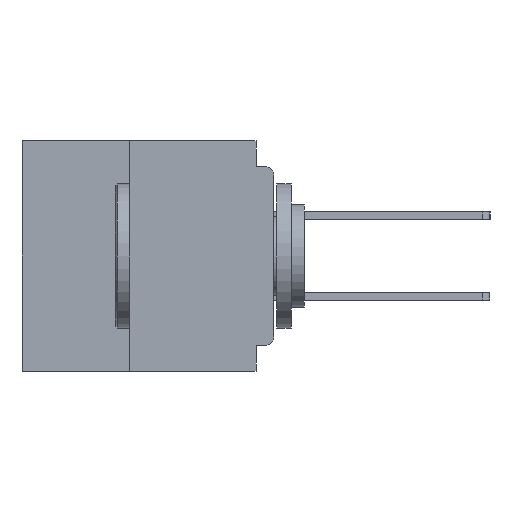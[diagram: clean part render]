
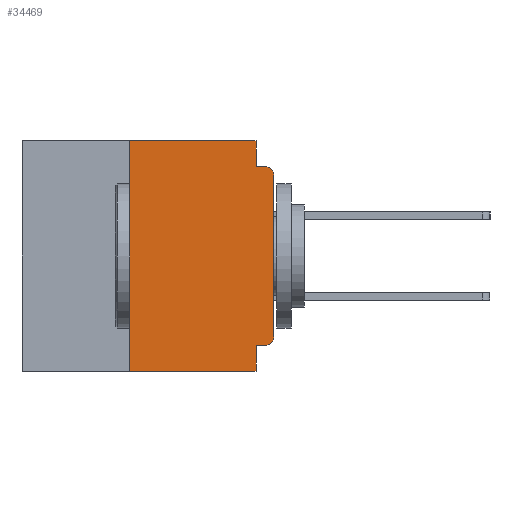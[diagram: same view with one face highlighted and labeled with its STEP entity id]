
A CAD part, left-side view. The second image highlights one B-rep face of the part: STEP entity #34469.
In plain terms, the highlighted planar face has unit normal (-1, 0, 0).
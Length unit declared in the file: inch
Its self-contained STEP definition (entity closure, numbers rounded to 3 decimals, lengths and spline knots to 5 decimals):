
#157 = ORIENTED_EDGE ( 'NONE', *, *, #12103, .T. ) ;
#930 = PLANE ( 'NONE',  #47290 ) ;
#1720 = LINE ( 'NONE', #28280, #22312 ) ;
#2714 = CARTESIAN_POINT ( 'NONE',  ( 0., 0.015, -0.34 ) ) ;
#3421 = CARTESIAN_POINT ( 'NONE',  ( 0., 0., -0.355 ) ) ;
#5037 = DIRECTION ( 'NONE',  ( 1., 0., 0. ) ) ;
#6052 = CARTESIAN_POINT ( 'NONE',  ( 0., 0.015, -0.06 ) ) ;
#6749 = EDGE_CURVE ( 'NONE', #33554, #48301, #14024, .T. ) ;
#6800 = DIRECTION ( 'NONE',  ( 0., 0., -1. ) ) ;
#7223 = CIRCLE ( 'NONE', #9165, 0.015 ) ;
#7630 = LINE ( 'NONE', #3421, #28279 ) ;
#8151 = CARTESIAN_POINT ( 'NONE',  ( 0., 0.031, -0.355 ) ) ;
#8238 = ORIENTED_EDGE ( 'NONE', *, *, #46837, .T. ) ;
#9165 = AXIS2_PLACEMENT_3D ( 'NONE', #6052, #34853, #10211 ) ;
#9646 = LINE ( 'NONE', #21950, #41076 ) ;
#10211 = DIRECTION ( 'NONE',  ( 0., 0., -1. ) ) ;
#10307 = EDGE_CURVE ( 'NONE', #15700, #12959, #27178, .T. ) ;
#10520 = CARTESIAN_POINT ( 'NONE',  ( 0., 0., 0. ) ) ;
#11860 = CARTESIAN_POINT ( 'NONE',  ( 0., 0.015, -0.045 ) ) ;
#12103 = EDGE_CURVE ( 'NONE', #51510, #29563, #7223, .T. ) ;
#12351 = CARTESIAN_POINT ( 'NONE',  ( 0., 0.25, 0. ) ) ;
#12959 = VERTEX_POINT ( 'NONE', #40966 ) ;
#13499 = LINE ( 'NONE', #20891, #43591 ) ;
#13823 = CARTESIAN_POINT ( 'NONE',  ( 0., 0.437, -0.4 ) ) ;
#13827 = EDGE_CURVE ( 'NONE', #42938, #48301, #9646, .T. ) ;
#13969 = LINE ( 'NONE', #10520, #33266 ) ;
#14024 = LINE ( 'NONE', #13823, #35861 ) ;
#14687 = DIRECTION ( 'NONE',  ( 0., 0., 1. ) ) ;
#15700 = VERTEX_POINT ( 'NONE', #17282 ) ;
#15825 = DIRECTION ( 'NONE',  ( 0., 1., 0. ) ) ;
#16198 = VECTOR ( 'NONE', #35724, 39.37008 ) ;
#17282 = CARTESIAN_POINT ( 'NONE',  ( 0., 0.031, 0. ) ) ;
#17295 = CARTESIAN_POINT ( 'NONE',  ( 0., 0.437, 0. ) ) ;
#17929 = DIRECTION ( 'NONE',  ( 0., -1., 0. ) ) ;
#18971 = ORIENTED_EDGE ( 'NONE', *, *, #45364, .F. ) ;
#19740 = CARTESIAN_POINT ( 'NONE',  ( 0., 0.031, -0.4 ) ) ;
#20891 = CARTESIAN_POINT ( 'NONE',  ( 0., 0., -0.045 ) ) ;
#21218 = AXIS2_PLACEMENT_3D ( 'NONE', #2714, #31515, #6800 ) ;
#21950 = CARTESIAN_POINT ( 'NONE',  ( 0., 0.031, -0.4 ) ) ;
#22312 = VECTOR ( 'NONE', #32408, 39.37008 ) ;
#24346 = EDGE_CURVE ( 'NONE', #32075, #15700, #1720, .T. ) ;
#25047 = DIRECTION ( 'NONE',  ( 0., -1., 0. ) ) ;
#25404 = CARTESIAN_POINT ( 'NONE',  ( 0., 0., -0.34 ) ) ;
#26085 = ORIENTED_EDGE ( 'NONE', *, *, #10307, .F. ) ;
#26274 = LINE ( 'NONE', #39543, #46629 ) ;
#26722 = CIRCLE ( 'NONE', #21218, 0.015 ) ;
#27002 = ORIENTED_EDGE ( 'NONE', *, *, #24346, .F. ) ;
#27017 = ORIENTED_EDGE ( 'NONE', *, *, #29402, .F. ) ;
#27178 = LINE ( 'NONE', #51826, #16198 ) ;
#28280 = CARTESIAN_POINT ( 'NONE',  ( 0., 0.437, 0. ) ) ;
#28279 = VECTOR ( 'NONE', #15825, 39.37008 ) ;
#29402 = EDGE_CURVE ( 'NONE', #33554, #32075, #26274, .T. ) ;
#29563 = VERTEX_POINT ( 'NONE', #11860 ) ;
#30284 = ORIENTED_EDGE ( 'NONE', *, *, #40615, .T. ) ;
#31515 = DIRECTION ( 'NONE',  ( -1., 0., 0. ) ) ;
#32075 = VERTEX_POINT ( 'NONE', #12351 ) ;
#32408 = DIRECTION ( 'NONE',  ( 0., -1., 0. ) ) ;
#32946 = EDGE_CURVE ( 'NONE', #40520, #42938, #7630, .T. ) ;
#33266 = VECTOR ( 'NONE', #14687, 39.37008 ) ;
#33554 = VERTEX_POINT ( 'NONE', #36058 ) ;
#33829 = DIRECTION ( 'NONE',  ( 0., 0., -1. ) ) ;
#34469 = ADVANCED_FACE ( 'NONE', ( #38323 ), #930, .F. ) ;
#34853 = DIRECTION ( 'NONE',  ( -1., 0., 0. ) ) ;
#34906 = CARTESIAN_POINT ( 'NONE',  ( 0., 0.015, -0.355 ) ) ;
#35234 = CARTESIAN_POINT ( 'NONE',  ( 0., 0., -0.06 ) ) ;
#35724 = DIRECTION ( 'NONE',  ( 0., 0., -1. ) ) ;
#35861 = VECTOR ( 'NONE', #17929, 39.37008 ) ;
#36002 = ORIENTED_EDGE ( 'NONE', *, *, #13827, .F. ) ;
#36058 = CARTESIAN_POINT ( 'NONE',  ( 0., 0.25, -0.4 ) ) ;
#38323 = FACE_OUTER_BOUND ( 'NONE', #38559, .T. ) ;
#38559 = EDGE_LOOP ( 'NONE', ( #8238, #157, #18971, #26085, #27002, #27017, #40355, #36002, #45187, #30284 ) ) ;
#39543 = CARTESIAN_POINT ( 'NONE',  ( 0., 0.25, -0.4 ) ) ;
#40355 = ORIENTED_EDGE ( 'NONE', *, *, #6749, .T. ) ;
#40520 = VERTEX_POINT ( 'NONE', #34906 ) ;
#40615 = EDGE_CURVE ( 'NONE', #40520, #52678, #26722, .T. ) ;
#40966 = CARTESIAN_POINT ( 'NONE',  ( 0., 0.031, -0.045 ) ) ;
#41076 = VECTOR ( 'NONE', #46375, 39.37008 ) ;
#42938 = VERTEX_POINT ( 'NONE', #8151 ) ;
#43591 = VECTOR ( 'NONE', #25047, 39.37008 ) ;
#43624 = DIRECTION ( 'NONE',  ( 0., 0., 1. ) ) ;
#45187 = ORIENTED_EDGE ( 'NONE', *, *, #32946, .F. ) ;
#45364 = EDGE_CURVE ( 'NONE', #12959, #29563, #13499, .T. ) ;
#46375 = DIRECTION ( 'NONE',  ( 0., 0., -1. ) ) ;
#46629 = VECTOR ( 'NONE', #43624, 39.37008 ) ;
#46837 = EDGE_CURVE ( 'NONE', #52678, #51510, #13969, .T. ) ;
#47290 = AXIS2_PLACEMENT_3D ( 'NONE', #17295, #5037, #33829 ) ;
#48301 = VERTEX_POINT ( 'NONE', #19740 ) ;
#51510 = VERTEX_POINT ( 'NONE', #35234 ) ;
#51826 = CARTESIAN_POINT ( 'NONE',  ( 0., 0.031, 0. ) ) ;
#52678 = VERTEX_POINT ( 'NONE', #25404 ) ;
